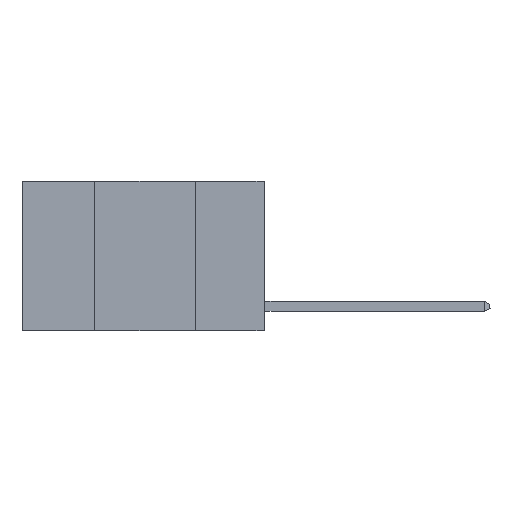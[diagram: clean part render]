
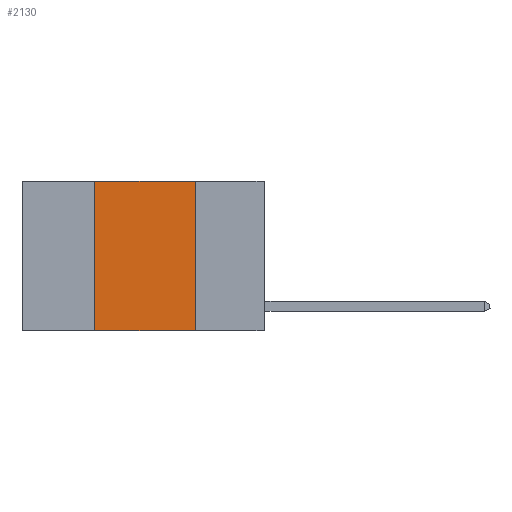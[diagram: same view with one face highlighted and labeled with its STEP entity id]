
A CAD part, left-side view. The second image highlights one B-rep face of the part: STEP entity #2130.
In plain terms, the highlighted planar face has unit normal (-1, 0, 0).
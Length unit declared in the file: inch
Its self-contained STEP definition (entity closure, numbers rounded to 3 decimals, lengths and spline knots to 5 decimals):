
#112 = DIRECTION ( 'NONE',  ( 1., 0., 0. ) ) ;
#800 = DIRECTION ( 'NONE',  ( 0., -1., 0. ) ) ;
#948 = CARTESIAN_POINT ( 'NONE',  ( 0., 0.42, 0. ) ) ;
#1280 = ORIENTED_EDGE ( 'NONE', *, *, #19555, .F. ) ;
#1854 = EDGE_CURVE ( 'NONE', #21195, #15393, #17829, .T. ) ;
#2130 = ADVANCED_FACE ( 'NONE', ( #15283 ), #7307, .F. ) ;
#3041 = VECTOR ( 'NONE', #16589, 39.37008 ) ;
#3636 = VECTOR ( 'NONE', #800, 39.37008 ) ;
#3769 = CARTESIAN_POINT ( 'NONE',  ( 0., 0.6, 0. ) ) ;
#4077 = LINE ( 'NONE', #5516, #5421 ) ;
#4106 = CARTESIAN_POINT ( 'NONE',  ( 0., 0.17, 0. ) ) ;
#5421 = VECTOR ( 'NONE', #15704, 39.37008 ) ;
#5516 = CARTESIAN_POINT ( 'NONE',  ( 0., 0.6, 0. ) ) ;
#5828 = EDGE_CURVE ( 'NONE', #8506, #6609, #4077, .T. ) ;
#6609 = VERTEX_POINT ( 'NONE', #4106 ) ;
#6868 = DIRECTION ( 'NONE',  ( 0., 0., -1. ) ) ;
#7307 = PLANE ( 'NONE',  #7798 ) ;
#7798 = AXIS2_PLACEMENT_3D ( 'NONE', #3769, #112, #6868 ) ;
#8506 = VERTEX_POINT ( 'NONE', #948 ) ;
#8596 = CARTESIAN_POINT ( 'NONE',  ( 0., 0.17, -0.37 ) ) ;
#9216 = EDGE_CURVE ( 'NONE', #6609, #15393, #20366, .T. ) ;
#9520 = LINE ( 'NONE', #16476, #3041 ) ;
#10346 = ORIENTED_EDGE ( 'NONE', *, *, #1854, .T. ) ;
#14299 = ORIENTED_EDGE ( 'NONE', *, *, #9216, .F. ) ;
#15200 = DIRECTION ( 'NONE',  ( 0., 0., -1. ) ) ;
#15283 = FACE_OUTER_BOUND ( 'NONE', #17872, .T. ) ;
#15393 = VERTEX_POINT ( 'NONE', #8596 ) ;
#15704 = DIRECTION ( 'NONE',  ( 0., -1., 0. ) ) ;
#16063 = CARTESIAN_POINT ( 'NONE',  ( 0., 0.6, -0.37 ) ) ;
#16476 = CARTESIAN_POINT ( 'NONE',  ( 0., 0.42, 0. ) ) ;
#16589 = DIRECTION ( 'NONE',  ( 0., 0., 1. ) ) ;
#17076 = CARTESIAN_POINT ( 'NONE',  ( 0., 0.17, 0. ) ) ;
#17829 = LINE ( 'NONE', #16063, #3636 ) ;
#17872 = EDGE_LOOP ( 'NONE', ( #14299, #18520, #1280, #10346 ) ) ;
#18520 = ORIENTED_EDGE ( 'NONE', *, *, #5828, .F. ) ;
#19555 = EDGE_CURVE ( 'NONE', #21195, #8506, #9520, .T. ) ;
#20366 = LINE ( 'NONE', #17076, #21348 ) ;
#21195 = VERTEX_POINT ( 'NONE', #21532 ) ;
#21348 = VECTOR ( 'NONE', #15200, 39.37008 ) ;
#21532 = CARTESIAN_POINT ( 'NONE',  ( 0., 0.42, -0.37 ) ) ;
